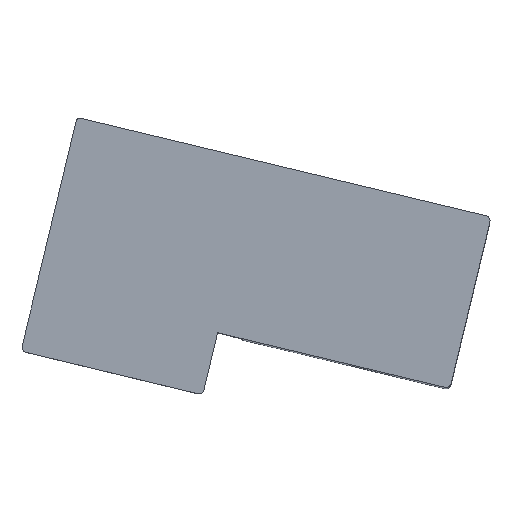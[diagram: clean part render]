
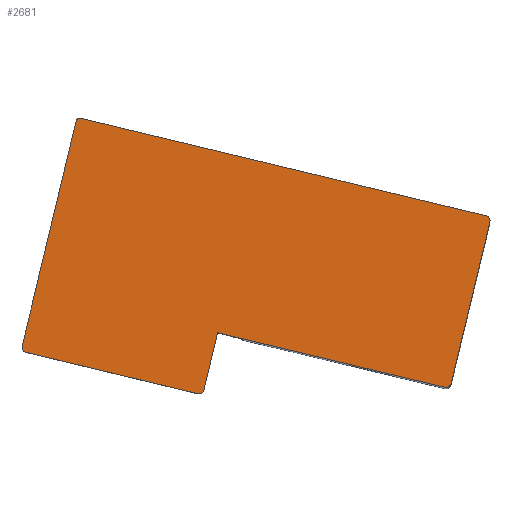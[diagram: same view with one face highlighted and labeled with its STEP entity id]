
A CAD part, top view. The second image highlights one B-rep face of the part: STEP entity #2681.
In plain terms, the highlighted planar face has unit normal (0, 0, 1).
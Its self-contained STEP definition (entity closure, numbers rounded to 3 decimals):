
#23 = ORIENTED_EDGE ( 'NONE', *, *, #1043, .F. ) ;
#38 = LINE ( 'NONE', #1762, #1280 ) ;
#49 = CARTESIAN_POINT ( 'NONE',  ( -23.663, -20.459, 19. ) ) ;
#120 = VERTEX_POINT ( 'NONE', #2273 ) ;
#157 = EDGE_CURVE ( 'NONE', #2139, #1125, #965, .T. ) ;
#171 = DIRECTION ( 'NONE',  ( 0., 0., 1. ) ) ;
#230 = CARTESIAN_POINT ( 'NONE',  ( -23.656, -20.401, 19. ) ) ;
#248 = ORIENTED_EDGE ( 'NONE', *, *, #610, .F. ) ;
#316 = VERTEX_POINT ( 'NONE', #1484 ) ;
#323 = EDGE_CURVE ( 'NONE', #2467, #420, #2332, .T. ) ;
#332 = AXIS2_PLACEMENT_3D ( 'NONE', #2292, #1909, #2099 ) ;
#366 = CARTESIAN_POINT ( 'NONE',  ( -43.052, -15.547, 19. ) ) ;
#412 = EDGE_CURVE ( 'NONE', #1021, #1419, #829, .T. ) ;
#420 = VERTEX_POINT ( 'NONE', #366 ) ;
#450 = ORIENTED_EDGE ( 'NONE', *, *, #2102, .F. ) ;
#459 = DIRECTION ( 'NONE',  ( 0., 0., -1. ) ) ;
#504 = VERTEX_POINT ( 'NONE', #2077 ) ;
#518 = VECTOR ( 'NONE', #2510, 1000. ) ;
#546 = CARTESIAN_POINT ( 'NONE',  ( -23.906, -20.401, 19. ) ) ;
#558 = CIRCLE ( 'NONE', #2132, 0.25 ) ;
#610 = EDGE_CURVE ( 'NONE', #1716, #755, #558, .T. ) ;
#617 = DIRECTION ( 'NONE',  ( -0.233, -0.972, 0. ) ) ;
#674 = CARTESIAN_POINT ( 'NONE',  ( -25.739, -28.035, 19. ) ) ;
#690 = DIRECTION ( 'NONE',  ( -0.972, 0.233, 0. ) ) ;
#718 = ORIENTED_EDGE ( 'NONE', *, *, #412, .T. ) ;
#755 = VERTEX_POINT ( 'NONE', #1584 ) ;
#766 = DIRECTION ( 'NONE',  ( -0.233, -0.972, 0. ) ) ;
#791 = DIRECTION ( 'NONE',  ( -0.999, -0.052, 0. ) ) ;
#805 = CARTESIAN_POINT ( 'NONE',  ( -45.61, -26.632, 19. ) ) ;
#829 = CIRCLE ( 'NONE', #2404, 0.25 ) ;
#912 = EDGE_CURVE ( 'NONE', #120, #316, #1855, .T. ) ;
#921 = EDGE_LOOP ( 'NONE', ( #1592, #2571, #1857, #248, #1700, #1789, #1617, #1636, #23, #450, #718, #1235, #2716 ) ) ;
#922 = EDGE_CURVE ( 'NONE', #2139, #2013, #1202, .T. ) ;
#965 = CIRCLE ( 'NONE', #2636, 0.25 ) ;
#983 = DIRECTION ( 'NONE',  ( 0., 0., -1. ) ) ;
#1021 = VERTEX_POINT ( 'NONE', #49 ) ;
#1041 = LINE ( 'NONE', #1908, #518 ) ;
#1043 = EDGE_CURVE ( 'NONE', #1586, #504, #2773, .T. ) ;
#1068 = DIRECTION ( 'NONE',  ( -0.972, 0.233, 0. ) ) ;
#1083 = CARTESIAN_POINT ( 'NONE',  ( -23.848, -20.158, 19. ) ) ;
#1125 = VERTEX_POINT ( 'NONE', #1618 ) ;
#1202 = LINE ( 'NONE', #1646, #2406 ) ;
#1213 = FACE_OUTER_BOUND ( 'NONE', #921, .T. ) ;
#1231 = VECTOR ( 'NONE', #766, 1000. ) ;
#1235 = ORIENTED_EDGE ( 'NONE', *, *, #2569, .T. ) ;
#1262 = DIRECTION ( 'NONE',  ( 0., 0., 1. ) ) ;
#1277 = AXIS2_PLACEMENT_3D ( 'NONE', #674, #459, #1578 ) ;
#1280 = VECTOR ( 'NONE', #690, 1000. ) ;
#1398 = CARTESIAN_POINT ( 'NONE',  ( -45.552, -26.389, 19. ) ) ;
#1406 = EDGE_CURVE ( 'NONE', #755, #316, #2260, .T. ) ;
#1410 = DIRECTION ( 'NONE',  ( 0., 0., -1. ) ) ;
#1419 = VERTEX_POINT ( 'NONE', #230 ) ;
#1427 = DIRECTION ( 'NONE',  ( 0.972, -0.233, 0. ) ) ;
#1468 = AXIS2_PLACEMENT_3D ( 'NONE', #2328, #1262, #2116 ) ;
#1472 = CARTESIAN_POINT ( 'NONE',  ( -24.579, -24.276, 19. ) ) ;
#1477 = EDGE_CURVE ( 'NONE', #504, #2013, #38, .T. ) ;
#1484 = CARTESIAN_POINT ( 'NONE',  ( -45.795, -26.331, 19. ) ) ;
#1578 = DIRECTION ( 'NONE',  ( 1., 0., 0. ) ) ;
#1584 = CARTESIAN_POINT ( 'NONE',  ( -45.802, -26.389, 19. ) ) ;
#1586 = VERTEX_POINT ( 'NONE', #1828 ) ;
#1592 = ORIENTED_EDGE ( 'NONE', *, *, #1683, .F. ) ;
#1601 = AXIS2_PLACEMENT_3D ( 'NONE', #2144, #2614, #1970 ) ;
#1617 = ORIENTED_EDGE ( 'NONE', *, *, #922, .T. ) ;
#1618 = CARTESIAN_POINT ( 'NONE',  ( -37.491, -28.581, 19. ) ) ;
#1636 = ORIENTED_EDGE ( 'NONE', *, *, #1477, .F. ) ;
#1639 = CARTESIAN_POINT ( 'NONE',  ( -36.542, -25.698, 19. ) ) ;
#1646 = CARTESIAN_POINT ( 'NONE',  ( -37.19, -28.397, 19. ) ) ;
#1683 = EDGE_CURVE ( 'NONE', #120, #420, #2401, .T. ) ;
#1700 = ORIENTED_EDGE ( 'NONE', *, *, #2704, .T. ) ;
#1716 = VERTEX_POINT ( 'NONE', #805 ) ;
#1723 = LINE ( 'NONE', #1472, #2635 ) ;
#1762 = CARTESIAN_POINT ( 'NONE',  ( -35.351, -25.984, 19. ) ) ;
#1789 = ORIENTED_EDGE ( 'NONE', *, *, #157, .F. ) ;
#1828 = CARTESIAN_POINT ( 'NONE',  ( -25.496, -28.093, 19. ) ) ;
#1835 = CARTESIAN_POINT ( 'NONE',  ( -37.433, -28.338, 19. ) ) ;
#1855 = LINE ( 'NONE', #2714, #1231 ) ;
#1857 = ORIENTED_EDGE ( 'NONE', *, *, #1406, .F. ) ;
#1878 = CARTESIAN_POINT ( 'NONE',  ( -23.848, -20.158, 19. ) ) ;
#1908 = CARTESIAN_POINT ( 'NONE',  ( -45.61, -26.632, 19. ) ) ;
#1909 = DIRECTION ( 'NONE',  ( 0., 0., -1. ) ) ;
#1920 = CARTESIAN_POINT ( 'NONE',  ( -37.19, -28.397, 19. ) ) ;
#1970 = DIRECTION ( 'NONE',  ( -0.233, -0.972, 0. ) ) ;
#2013 = VERTEX_POINT ( 'NONE', #1639 ) ;
#2040 = VECTOR ( 'NONE', #1068, 1000. ) ;
#2077 = CARTESIAN_POINT ( 'NONE',  ( -25.797, -28.278, 19. ) ) ;
#2079 = DIRECTION ( 'NONE',  ( -0.233, -0.972, 0. ) ) ;
#2098 = CARTESIAN_POINT ( 'NONE',  ( -23.895, -14.491, 19. ) ) ;
#2099 = DIRECTION ( 'NONE',  ( -0.972, 0.233, 0. ) ) ;
#2102 = EDGE_CURVE ( 'NONE', #1021, #1586, #1723, .T. ) ;
#2112 = PLANE ( 'NONE',  #2590 ) ;
#2116 = DIRECTION ( 'NONE',  ( 1., 0., 0. ) ) ;
#2132 = AXIS2_PLACEMENT_3D ( 'NONE', #1398, #1410, #617 ) ;
#2139 = VERTEX_POINT ( 'NONE', #1920 ) ;
#2144 = CARTESIAN_POINT ( 'NONE',  ( -45.552, -26.389, 19. ) ) ;
#2260 = CIRCLE ( 'NONE', #1601, 0.25 ) ;
#2263 = DIRECTION ( 'NONE',  ( 0., 0., 1. ) ) ;
#2273 = CARTESIAN_POINT ( 'NONE',  ( -43.233, -15.658, 19. ) ) ;
#2274 = DIRECTION ( 'NONE',  ( 1., 0., 0. ) ) ;
#2281 = DIRECTION ( 'NONE',  ( 0.233, 0.972, 0. ) ) ;
#2292 = CARTESIAN_POINT ( 'NONE',  ( -43.087, -15.693, 19. ) ) ;
#2328 = CARTESIAN_POINT ( 'NONE',  ( -23.906, -20.401, 19. ) ) ;
#2332 = LINE ( 'NONE', #1083, #2040 ) ;
#2362 = CIRCLE ( 'NONE', #1468, 0.25 ) ;
#2401 = CIRCLE ( 'NONE', #332, 0.15 ) ;
#2404 = AXIS2_PLACEMENT_3D ( 'NONE', #546, #2263, #2274 ) ;
#2406 = VECTOR ( 'NONE', #2281, 1000. ) ;
#2467 = VERTEX_POINT ( 'NONE', #1878 ) ;
#2510 = DIRECTION ( 'NONE',  ( 0.972, -0.233, 0. ) ) ;
#2569 = EDGE_CURVE ( 'NONE', #1419, #2467, #2362, .T. ) ;
#2571 = ORIENTED_EDGE ( 'NONE', *, *, #912, .T. ) ;
#2590 = AXIS2_PLACEMENT_3D ( 'NONE', #2098, #171, #791 ) ;
#2614 = DIRECTION ( 'NONE',  ( 0., 0., -1. ) ) ;
#2635 = VECTOR ( 'NONE', #2079, 1000. ) ;
#2636 = AXIS2_PLACEMENT_3D ( 'NONE', #1835, #983, #1427 ) ;
#2681 = ADVANCED_FACE ( 'NONE', ( #1213 ), #2112, .T. ) ;
#2704 = EDGE_CURVE ( 'NONE', #1716, #1125, #1041, .T. ) ;
#2714 = CARTESIAN_POINT ( 'NONE',  ( -43.233, -15.658, 19. ) ) ;
#2716 = ORIENTED_EDGE ( 'NONE', *, *, #323, .T. ) ;
#2773 = CIRCLE ( 'NONE', #1277, 0.25 ) ;
